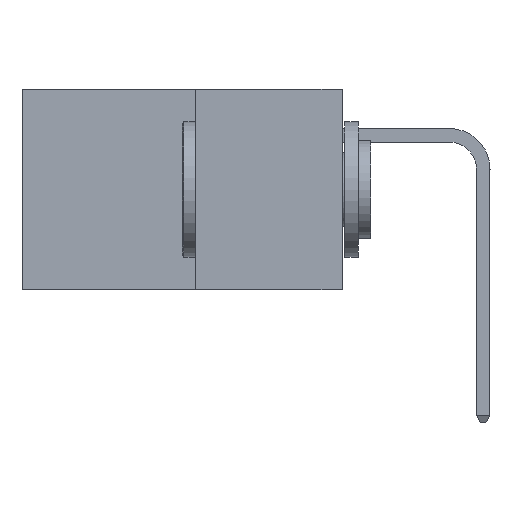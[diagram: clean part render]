
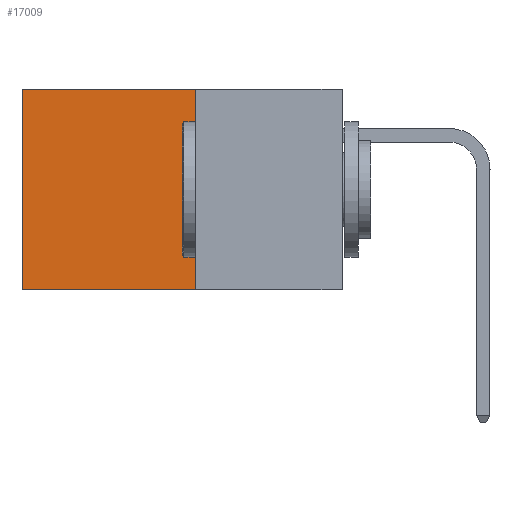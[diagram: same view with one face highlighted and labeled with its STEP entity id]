
A CAD part, left-side view. The second image highlights one B-rep face of the part: STEP entity #17009.
In plain terms, the highlighted planar face has unit normal (-1, 0, 0).
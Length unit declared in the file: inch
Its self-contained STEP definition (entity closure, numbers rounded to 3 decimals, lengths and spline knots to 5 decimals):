
#87 = CARTESIAN_POINT ( 'NONE',  ( 0.277, 0.27, 0. ) ) ;
#1915 = VECTOR ( 'NONE', #16160, 39.37008 ) ;
#3339 = VERTEX_POINT ( 'NONE', #18083 ) ;
#3652 = DIRECTION ( 'NONE',  ( 0., 0., -1. ) ) ;
#5082 = VECTOR ( 'NONE', #11338, 39.37008 ) ;
#5649 = LINE ( 'NONE', #9577, #5082 ) ;
#5960 = VERTEX_POINT ( 'NONE', #11179 ) ;
#6766 = LINE ( 'NONE', #87, #1915 ) ;
#7821 = CARTESIAN_POINT ( 'NONE',  ( 0.277, 0.27, -0.37 ) ) ;
#8003 = EDGE_CURVE ( 'NONE', #5960, #9409, #5649, .T. ) ;
#8061 = VECTOR ( 'NONE', #14865, 39.37008 ) ;
#8388 = EDGE_CURVE ( 'NONE', #5960, #18037, #6766, .T. ) ;
#8526 = ORIENTED_EDGE ( 'NONE', *, *, #17867, .F. ) ;
#9200 = ORIENTED_EDGE ( 'NONE', *, *, #8003, .F. ) ;
#9409 = VERTEX_POINT ( 'NONE', #10497 ) ;
#9577 = CARTESIAN_POINT ( 'NONE',  ( 0.277, 0.27, -0.37 ) ) ;
#10441 = EDGE_LOOP ( 'NONE', ( #13164, #8526, #9200, #14625 ) ) ;
#10497 = CARTESIAN_POINT ( 'NONE',  ( 0.277, 0.27, -0.37 ) ) ;
#11179 = CARTESIAN_POINT ( 'NONE',  ( 0.277, 0.27, 0. ) ) ;
#11239 = VECTOR ( 'NONE', #13519, 39.37008 ) ;
#11338 = DIRECTION ( 'NONE',  ( 0., 0., -1. ) ) ;
#12585 = PLANE ( 'NONE',  #22026 ) ;
#13164 = ORIENTED_EDGE ( 'NONE', *, *, #21358, .T. ) ;
#13519 = DIRECTION ( 'NONE',  ( 0., 0., -1. ) ) ;
#13562 = CARTESIAN_POINT ( 'NONE',  ( 0.277, 0.59, 0. ) ) ;
#13723 = CARTESIAN_POINT ( 'NONE',  ( 0.277, 0.27, -0.37 ) ) ;
#14339 = DIRECTION ( 'NONE',  ( 1., 0., 0. ) ) ;
#14625 = ORIENTED_EDGE ( 'NONE', *, *, #8388, .T. ) ;
#14865 = DIRECTION ( 'NONE',  ( 0., 1., 0. ) ) ;
#15118 = CARTESIAN_POINT ( 'NONE',  ( 0.277, 0.59, -0.37 ) ) ;
#15860 = LINE ( 'NONE', #15118, #11239 ) ;
#16160 = DIRECTION ( 'NONE',  ( 0., 1., 0. ) ) ;
#17009 = ADVANCED_FACE ( 'NONE', ( #17386 ), #12585, .F. ) ;
#17342 = LINE ( 'NONE', #7821, #8061 ) ;
#17386 = FACE_OUTER_BOUND ( 'NONE', #10441, .T. ) ;
#17867 = EDGE_CURVE ( 'NONE', #9409, #3339, #17342, .T. ) ;
#18037 = VERTEX_POINT ( 'NONE', #13562 ) ;
#18083 = CARTESIAN_POINT ( 'NONE',  ( 0.277, 0.59, -0.37 ) ) ;
#21358 = EDGE_CURVE ( 'NONE', #18037, #3339, #15860, .T. ) ;
#22026 = AXIS2_PLACEMENT_3D ( 'NONE', #13723, #14339, #3652 ) ;
